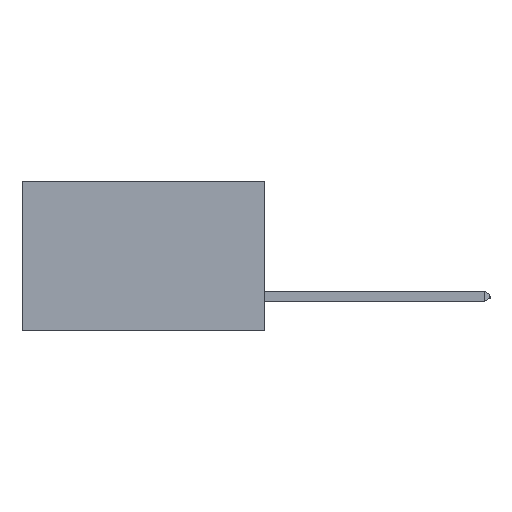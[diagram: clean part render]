
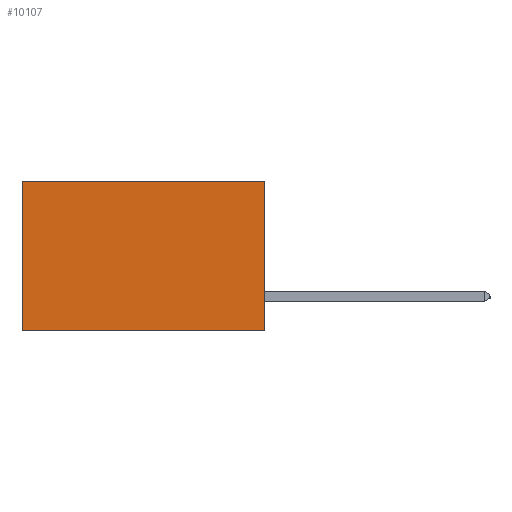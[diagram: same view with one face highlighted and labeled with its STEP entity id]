
A CAD part, left-side view. The second image highlights one B-rep face of the part: STEP entity #10107.
In plain terms, the highlighted planar face has unit normal (-1, 0, 0).
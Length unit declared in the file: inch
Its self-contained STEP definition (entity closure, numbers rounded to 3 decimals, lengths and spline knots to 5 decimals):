
#1190 = CARTESIAN_POINT ( 'NONE',  ( 0.298, 0., -0.37 ) ) ;
#1510 = LINE ( 'NONE', #5451, #17447 ) ;
#1965 = ORIENTED_EDGE ( 'NONE', *, *, #2591, .T. ) ;
#2139 = CARTESIAN_POINT ( 'NONE',  ( 0.298, 0., -0.37 ) ) ;
#2591 = EDGE_CURVE ( 'NONE', #13742, #17575, #8407, .T. ) ;
#2881 = LINE ( 'NONE', #2139, #3402 ) ;
#3402 = VECTOR ( 'NONE', #13451, 39.37008 ) ;
#3824 = CARTESIAN_POINT ( 'NONE',  ( 0.298, 0., 0. ) ) ;
#5451 = CARTESIAN_POINT ( 'NONE',  ( 0.298, 0., 0. ) ) ;
#5486 = DIRECTION ( 'NONE',  ( 0., 0., -1. ) ) ;
#7078 = DIRECTION ( 'NONE',  ( 0., 1., 0. ) ) ;
#8407 = LINE ( 'NONE', #15003, #8936 ) ;
#8476 = ORIENTED_EDGE ( 'NONE', *, *, #20433, .T. ) ;
#8929 = DIRECTION ( 'NONE',  ( 1., 0., 0. ) ) ;
#8936 = VECTOR ( 'NONE', #17093, 39.37008 ) ;
#9298 = CARTESIAN_POINT ( 'NONE',  ( 0.298, 0.6, -0.37 ) ) ;
#9692 = VECTOR ( 'NONE', #5486, 39.37008 ) ;
#10107 = ADVANCED_FACE ( 'NONE', ( #18606 ), #10448, .F. ) ;
#10199 = LINE ( 'NONE', #3824, #9692 ) ;
#10341 = AXIS2_PLACEMENT_3D ( 'NONE', #18123, #8929, #19636 ) ;
#10448 = PLANE ( 'NONE',  #10341 ) ;
#11250 = EDGE_CURVE ( 'NONE', #19379, #12564, #10199, .T. ) ;
#11298 = ORIENTED_EDGE ( 'NONE', *, *, #12287, .F. ) ;
#12287 = EDGE_CURVE ( 'NONE', #12564, #17575, #2881, .T. ) ;
#12564 = VERTEX_POINT ( 'NONE', #1190 ) ;
#13451 = DIRECTION ( 'NONE',  ( 0., 1., 0. ) ) ;
#13742 = VERTEX_POINT ( 'NONE', #14139 ) ;
#14139 = CARTESIAN_POINT ( 'NONE',  ( 0.298, 0.6, 0. ) ) ;
#15003 = CARTESIAN_POINT ( 'NONE',  ( 0.298, 0.6, 0. ) ) ;
#17093 = DIRECTION ( 'NONE',  ( 0., 0., -1. ) ) ;
#17292 = ORIENTED_EDGE ( 'NONE', *, *, #11250, .F. ) ;
#17447 = VECTOR ( 'NONE', #7078, 39.37008 ) ;
#17575 = VERTEX_POINT ( 'NONE', #9298 ) ;
#18123 = CARTESIAN_POINT ( 'NONE',  ( 0.298, 0., 0. ) ) ;
#18480 = CARTESIAN_POINT ( 'NONE',  ( 0.298, 0., 0. ) ) ;
#18606 = FACE_OUTER_BOUND ( 'NONE', #19042, .T. ) ;
#19042 = EDGE_LOOP ( 'NONE', ( #1965, #11298, #17292, #8476 ) ) ;
#19379 = VERTEX_POINT ( 'NONE', #18480 ) ;
#19636 = DIRECTION ( 'NONE',  ( 0., 0., -1. ) ) ;
#20433 = EDGE_CURVE ( 'NONE', #19379, #13742, #1510, .T. ) ;
